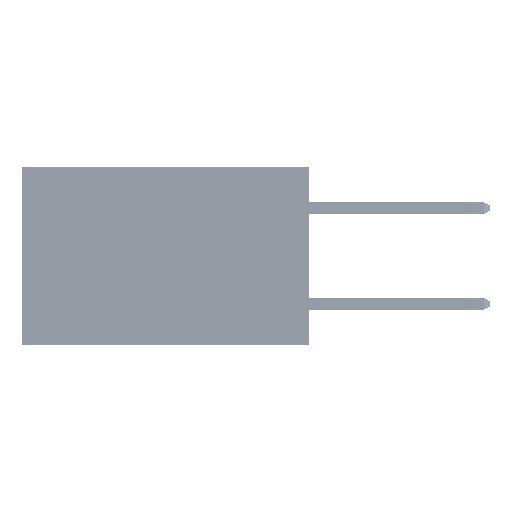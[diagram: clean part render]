
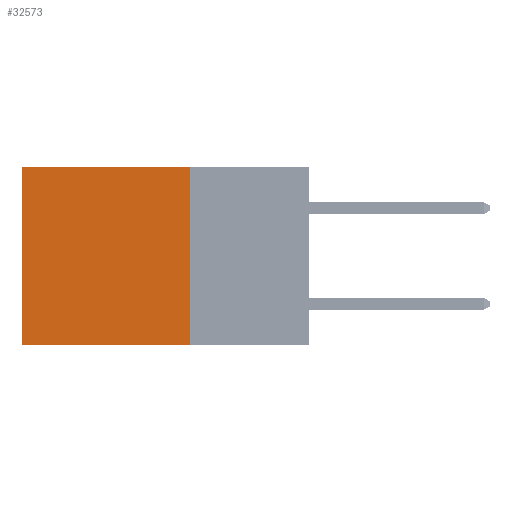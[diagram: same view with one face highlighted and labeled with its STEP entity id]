
A CAD part, left-side view. The second image highlights one B-rep face of the part: STEP entity #32573.
In plain terms, the highlighted planar face has unit normal (-1, 0, 0).
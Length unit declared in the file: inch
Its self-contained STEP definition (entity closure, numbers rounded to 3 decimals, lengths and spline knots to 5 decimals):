
#1301 = VECTOR ( 'NONE', #41960, 39.37008 ) ;
#2852 = EDGE_CURVE ( 'NONE', #11269, #27151, #4625, .T. ) ;
#3665 = CARTESIAN_POINT ( 'NONE',  ( 0.2875, 0.6, -0.37 ) ) ;
#4159 = DIRECTION ( 'NONE',  ( 0., 0., -1. ) ) ;
#4332 = DIRECTION ( 'NONE',  ( 0., 0., -1. ) ) ;
#4625 = LINE ( 'NONE', #14521, #35963 ) ;
#4687 = ORIENTED_EDGE ( 'NONE', *, *, #27272, .F. ) ;
#6297 = DIRECTION ( 'NONE',  ( 0., 1., 0. ) ) ;
#6777 = DIRECTION ( 'NONE',  ( 0., 1., 0. ) ) ;
#8345 = DIRECTION ( 'NONE',  ( 1., 0., 0. ) ) ;
#8655 = CARTESIAN_POINT ( 'NONE',  ( 0.2875, 0.25, -0.37 ) ) ;
#9410 = FACE_OUTER_BOUND ( 'NONE', #27687, .T. ) ;
#9544 = VECTOR ( 'NONE', #4332, 39.37008 ) ;
#9723 = LINE ( 'NONE', #26290, #25453 ) ;
#11269 = VERTEX_POINT ( 'NONE', #44670 ) ;
#12083 = ORIENTED_EDGE ( 'NONE', *, *, #2852, .T. ) ;
#12391 = ORIENTED_EDGE ( 'NONE', *, *, #18511, .F. ) ;
#14076 = EDGE_CURVE ( 'NONE', #27151, #28236, #35911, .T. ) ;
#14521 = CARTESIAN_POINT ( 'NONE',  ( 0.2875, 0.25, 0. ) ) ;
#14636 = VERTEX_POINT ( 'NONE', #8655 ) ;
#18511 = EDGE_CURVE ( 'NONE', #14636, #28236, #9723, .T. ) ;
#19382 = CARTESIAN_POINT ( 'NONE',  ( 0.2875, 0.6, 0. ) ) ;
#21996 = CARTESIAN_POINT ( 'NONE',  ( 0.2875, 0.25, 0. ) ) ;
#24525 = LINE ( 'NONE', #21996, #1301 ) ;
#25453 = VECTOR ( 'NONE', #6297, 39.37008 ) ;
#26290 = CARTESIAN_POINT ( 'NONE',  ( 0.2875, 0.25, -0.37 ) ) ;
#27151 = VERTEX_POINT ( 'NONE', #49502 ) ;
#27272 = EDGE_CURVE ( 'NONE', #11269, #14636, #24525, .T. ) ;
#27687 = EDGE_LOOP ( 'NONE', ( #29038, #12391, #4687, #12083 ) ) ;
#28236 = VERTEX_POINT ( 'NONE', #3665 ) ;
#29038 = ORIENTED_EDGE ( 'NONE', *, *, #14076, .T. ) ;
#32573 = ADVANCED_FACE ( 'NONE', ( #9410 ), #47462, .F. ) ;
#35911 = LINE ( 'NONE', #19382, #9544 ) ;
#35963 = VECTOR ( 'NONE', #6777, 39.37008 ) ;
#39720 = CARTESIAN_POINT ( 'NONE',  ( 0.2875, 0.25, 0. ) ) ;
#41960 = DIRECTION ( 'NONE',  ( 0., 0., -1. ) ) ;
#42952 = AXIS2_PLACEMENT_3D ( 'NONE', #39720, #8345, #4159 ) ;
#44670 = CARTESIAN_POINT ( 'NONE',  ( 0.2875, 0.25, 0. ) ) ;
#47462 = PLANE ( 'NONE',  #42952 ) ;
#49502 = CARTESIAN_POINT ( 'NONE',  ( 0.2875, 0.6, 0. ) ) ;
